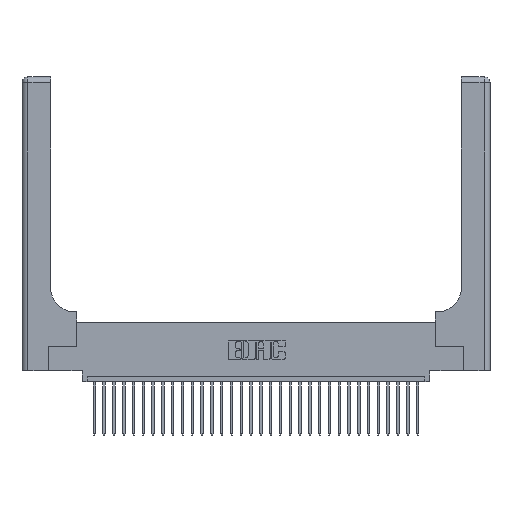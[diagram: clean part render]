
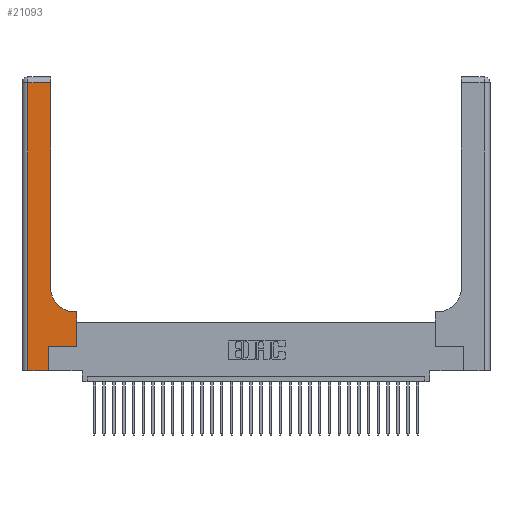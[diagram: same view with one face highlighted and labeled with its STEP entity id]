
A CAD part, top view. The second image highlights one B-rep face of the part: STEP entity #21093.
In plain terms, the highlighted planar face has unit normal (0, 0, 1).
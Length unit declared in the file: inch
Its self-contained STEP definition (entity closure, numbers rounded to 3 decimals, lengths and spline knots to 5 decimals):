
#977 = VERTEX_POINT ( 'NONE', #14571 ) ;
#1056 = CARTESIAN_POINT ( 'NONE',  ( 0.5415, 0.6, 0.37 ) ) ;
#1396 = VERTEX_POINT ( 'NONE', #3198 ) ;
#1419 = LINE ( 'NONE', #6234, #1782 ) ;
#1468 = VECTOR ( 'NONE', #16392, 39.37008 ) ;
#1480 = VERTEX_POINT ( 'NONE', #4048 ) ;
#1534 = CARTESIAN_POINT ( 'NONE',  ( 0.06, 3., 0.37 ) ) ;
#1782 = VECTOR ( 'NONE', #8304, 39.37008 ) ;
#2148 = EDGE_CURVE ( 'NONE', #7688, #27270, #22287, .T. ) ;
#2542 = DIRECTION ( 'NONE',  ( 0., 1., 0. ) ) ;
#3198 = CARTESIAN_POINT ( 'NONE',  ( 0.06, 0., 0.37 ) ) ;
#4048 = CARTESIAN_POINT ( 'NONE',  ( 0.269, 0.25, 0.37 ) ) ;
#4394 = VERTEX_POINT ( 'NONE', #21284 ) ;
#4403 = ORIENTED_EDGE ( 'NONE', *, *, #8567, .T. ) ;
#4692 = EDGE_CURVE ( 'NONE', #977, #5824, #1419, .T. ) ;
#4747 = CARTESIAN_POINT ( 'NONE',  ( 0.5415, 0.85, 0.37 ) ) ;
#5824 = VERTEX_POINT ( 'NONE', #31367 ) ;
#6234 = CARTESIAN_POINT ( 'NONE',  ( 0., 2.94, 0.37 ) ) ;
#6324 = PLANE ( 'NONE',  #23506 ) ;
#6352 = ORIENTED_EDGE ( 'NONE', *, *, #11403, .T. ) ;
#6539 = DIRECTION ( 'NONE',  ( 0., 0., -1. ) ) ;
#6730 = CARTESIAN_POINT ( 'NONE',  ( 0.269, 0., 0.37 ) ) ;
#6874 = LINE ( 'NONE', #21580, #1468 ) ;
#7195 = ORIENTED_EDGE ( 'NONE', *, *, #2148, .T. ) ;
#7422 = CARTESIAN_POINT ( 'NONE',  ( 0.2915, 3., 0.37 ) ) ;
#7688 = VERTEX_POINT ( 'NONE', #8702 ) ;
#7772 = CARTESIAN_POINT ( 'NONE',  ( 0.2915, 0.85, 0.37 ) ) ;
#8304 = DIRECTION ( 'NONE',  ( -1., 0., 0. ) ) ;
#8567 = EDGE_CURVE ( 'NONE', #1480, #4394, #12430, .T. ) ;
#8702 = CARTESIAN_POINT ( 'NONE',  ( 0.5585, 0.6, 0.37 ) ) ;
#9770 = DIRECTION ( 'NONE',  ( 1., 0., 0. ) ) ;
#11042 = CARTESIAN_POINT ( 'NONE',  ( 0.269, 0., 0.37 ) ) ;
#11403 = EDGE_CURVE ( 'NONE', #24976, #1480, #16193, .T. ) ;
#11607 = CARTESIAN_POINT ( 'NONE',  ( 0.2915, 0.6, 0.37 ) ) ;
#12430 = LINE ( 'NONE', #15396, #18991 ) ;
#12578 = EDGE_LOOP ( 'NONE', ( #22995, #25357, #29641, #27374, #6352, #4403, #28148, #7195, #27963 ) ) ;
#13599 = DIRECTION ( 'NONE',  ( 0., 1., 0. ) ) ;
#14034 = EDGE_CURVE ( 'NONE', #4394, #7688, #20669, .T. ) ;
#14571 = CARTESIAN_POINT ( 'NONE',  ( 0.2915, 2.94, 0.37 ) ) ;
#15396 = CARTESIAN_POINT ( 'NONE',  ( 0.269, 0.25, 0.37 ) ) ;
#16193 = LINE ( 'NONE', #6730, #23188 ) ;
#16392 = DIRECTION ( 'NONE',  ( 1., 0., 0. ) ) ;
#16429 = DIRECTION ( 'NONE',  ( -1., 0., 0. ) ) ;
#16788 = EDGE_CURVE ( 'NONE', #27270, #29225, #25021, .T. ) ;
#18543 = DIRECTION ( 'NONE',  ( 1., 0., 0. ) ) ;
#18991 = VECTOR ( 'NONE', #18543, 39.37008 ) ;
#19809 = VECTOR ( 'NONE', #2542, 39.37008 ) ;
#20090 = FACE_OUTER_BOUND ( 'NONE', #12578, .T. ) ;
#20241 = VECTOR ( 'NONE', #24717, 39.37008 ) ;
#20497 = AXIS2_PLACEMENT_3D ( 'NONE', #4747, #22107, #9770 ) ;
#20669 = LINE ( 'NONE', #28425, #25302 ) ;
#21093 = ADVANCED_FACE ( 'NONE', ( #20090 ), #6324, .F. ) ;
#21284 = CARTESIAN_POINT ( 'NONE',  ( 0.5585, 0.25, 0.37 ) ) ;
#21375 = LINE ( 'NONE', #7422, #19809 ) ;
#21580 = CARTESIAN_POINT ( 'NONE',  ( 0., 0., 0.37 ) ) ;
#21770 = EDGE_CURVE ( 'NONE', #1396, #24976, #6874, .T. ) ;
#22107 = DIRECTION ( 'NONE',  ( 0., 0., -1. ) ) ;
#22287 = LINE ( 'NONE', #11607, #26528 ) ;
#22995 = ORIENTED_EDGE ( 'NONE', *, *, #31938, .T. ) ;
#23188 = VECTOR ( 'NONE', #29019, 39.37008 ) ;
#23373 = LINE ( 'NONE', #1534, #20241 ) ;
#23506 = AXIS2_PLACEMENT_3D ( 'NONE', #23684, #6539, #16429 ) ;
#23684 = CARTESIAN_POINT ( 'NONE',  ( 0., 3., 0.37 ) ) ;
#24717 = DIRECTION ( 'NONE',  ( 0., -1., 0. ) ) ;
#24976 = VERTEX_POINT ( 'NONE', #11042 ) ;
#25021 = CIRCLE ( 'NONE', #20497, 0.25 ) ;
#25302 = VECTOR ( 'NONE', #13599, 39.37008 ) ;
#25357 = ORIENTED_EDGE ( 'NONE', *, *, #4692, .T. ) ;
#26528 = VECTOR ( 'NONE', #28872, 39.37008 ) ;
#27270 = VERTEX_POINT ( 'NONE', #1056 ) ;
#27374 = ORIENTED_EDGE ( 'NONE', *, *, #21770, .T. ) ;
#27963 = ORIENTED_EDGE ( 'NONE', *, *, #16788, .T. ) ;
#28148 = ORIENTED_EDGE ( 'NONE', *, *, #14034, .T. ) ;
#28425 = CARTESIAN_POINT ( 'NONE',  ( 0.5585, 0.25, 0.37 ) ) ;
#28872 = DIRECTION ( 'NONE',  ( -1., 0., 0. ) ) ;
#29019 = DIRECTION ( 'NONE',  ( 0., 1., 0. ) ) ;
#29225 = VERTEX_POINT ( 'NONE', #7772 ) ;
#29641 = ORIENTED_EDGE ( 'NONE', *, *, #31276, .T. ) ;
#31276 = EDGE_CURVE ( 'NONE', #5824, #1396, #23373, .T. ) ;
#31367 = CARTESIAN_POINT ( 'NONE',  ( 0.06, 2.94, 0.37 ) ) ;
#31938 = EDGE_CURVE ( 'NONE', #29225, #977, #21375, .T. ) ;
